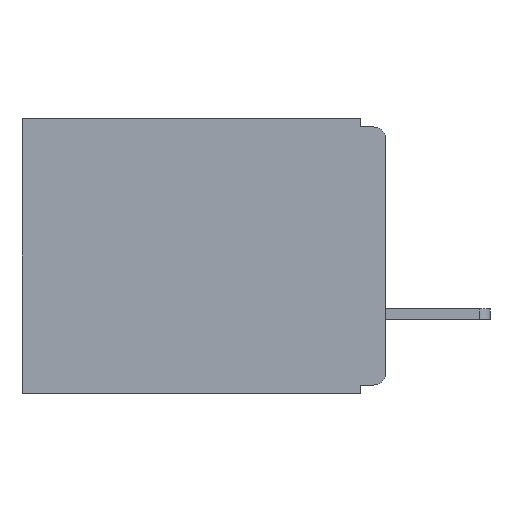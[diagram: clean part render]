
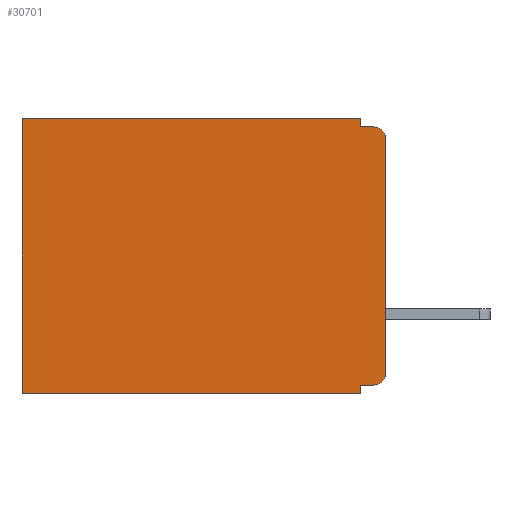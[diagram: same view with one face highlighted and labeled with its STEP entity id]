
A CAD part, left-side view. The second image highlights one B-rep face of the part: STEP entity #30701.
In plain terms, the highlighted planar face has unit normal (-1, 0, 0).
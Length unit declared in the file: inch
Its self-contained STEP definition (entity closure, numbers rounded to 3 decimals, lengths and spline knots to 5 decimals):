
#264 = VERTEX_POINT ( 'NONE', #18152 ) ;
#410 = LINE ( 'NONE', #27130, #25650 ) ;
#534 = ORIENTED_EDGE ( 'NONE', *, *, #4870, .F. ) ;
#1173 = FACE_OUTER_BOUND ( 'NONE', #26101, .T. ) ;
#1331 = ORIENTED_EDGE ( 'NONE', *, *, #5463, .F. ) ;
#1792 = AXIS2_PLACEMENT_3D ( 'NONE', #12589, #29337, #15085 ) ;
#1932 = VERTEX_POINT ( 'NONE', #24491 ) ;
#1987 = VERTEX_POINT ( 'NONE', #24394 ) ;
#2111 = LINE ( 'NONE', #21609, #7904 ) ;
#2284 = ORIENTED_EDGE ( 'NONE', *, *, #25020, .T. ) ;
#2735 = VECTOR ( 'NONE', #19983, 39.37008 ) ;
#3111 = ORIENTED_EDGE ( 'NONE', *, *, #28612, .T. ) ;
#3761 = DIRECTION ( 'NONE',  ( 0., 0., -1. ) ) ;
#3838 = ORIENTED_EDGE ( 'NONE', *, *, #11249, .F. ) ;
#4196 = DIRECTION ( 'NONE',  ( 0., -1., 0. ) ) ;
#4428 = DIRECTION ( 'NONE',  ( 0., 0., -1. ) ) ;
#4479 = CARTESIAN_POINT ( 'NONE',  ( 0.3, 0., -0.305 ) ) ;
#4870 = EDGE_CURVE ( 'NONE', #17214, #27444, #29079, .T. ) ;
#5152 = CARTESIAN_POINT ( 'NONE',  ( 0.3, 0., -0.32 ) ) ;
#5463 = EDGE_CURVE ( 'NONE', #6183, #6926, #17572, .T. ) ;
#5671 = CARTESIAN_POINT ( 'NONE',  ( 0.3, 0.437, -0.33 ) ) ;
#5699 = ORIENTED_EDGE ( 'NONE', *, *, #7581, .F. ) ;
#6183 = VERTEX_POINT ( 'NONE', #15034 ) ;
#6699 = ORIENTED_EDGE ( 'NONE', *, *, #14913, .T. ) ;
#6926 = VERTEX_POINT ( 'NONE', #8152 ) ;
#7234 = ORIENTED_EDGE ( 'NONE', *, *, #10860, .F. ) ;
#7368 = EDGE_CURVE ( 'NONE', #17056, #27444, #7726, .T. ) ;
#7581 = EDGE_CURVE ( 'NONE', #1987, #264, #21901, .T. ) ;
#7591 = ORIENTED_EDGE ( 'NONE', *, *, #11203, .F. ) ;
#7726 = CIRCLE ( 'NONE', #21765, 0.015 ) ;
#7904 = VECTOR ( 'NONE', #9402, 39.37008 ) ;
#8152 = CARTESIAN_POINT ( 'NONE',  ( 0.3, 0.015, -0.01 ) ) ;
#8206 = ORIENTED_EDGE ( 'NONE', *, *, #7368, .T. ) ;
#8566 = LINE ( 'NONE', #5152, #2735 ) ;
#9402 = DIRECTION ( 'NONE',  ( 0., 1., 0. ) ) ;
#10323 = VERTEX_POINT ( 'NONE', #28539 ) ;
#10860 = EDGE_CURVE ( 'NONE', #1932, #1987, #24191, .T. ) ;
#10916 = DIRECTION ( 'NONE',  ( 0., 0., -1. ) ) ;
#11162 = DIRECTION ( 'NONE',  ( -1., 0., 0. ) ) ;
#11203 = EDGE_CURVE ( 'NONE', #17056, #1932, #8566, .T. ) ;
#11249 = EDGE_CURVE ( 'NONE', #25748, #6183, #410, .T. ) ;
#11384 = CARTESIAN_POINT ( 'NONE',  ( 0.3, 0.015, -0.305 ) ) ;
#12258 = CARTESIAN_POINT ( 'NONE',  ( 0.3, 0.015, -0.32 ) ) ;
#12589 = CARTESIAN_POINT ( 'NONE',  ( 0.3, 0.015, -0.025 ) ) ;
#12863 = CARTESIAN_POINT ( 'NONE',  ( 0.3, 0.031, 0. ) ) ;
#12900 = CARTESIAN_POINT ( 'NONE',  ( 0.3, 0., -0.025 ) ) ;
#14736 = VECTOR ( 'NONE', #30109, 39.37008 ) ;
#14913 = EDGE_CURVE ( 'NONE', #10323, #264, #30010, .T. ) ;
#15034 = CARTESIAN_POINT ( 'NONE',  ( 0.3, 0.031, -0.01 ) ) ;
#15085 = DIRECTION ( 'NONE',  ( 0., 0., -1. ) ) ;
#16164 = CARTESIAN_POINT ( 'NONE',  ( 0.3, 0.031, -0.33 ) ) ;
#16817 = VECTOR ( 'NONE', #4196, 39.37008 ) ;
#17056 = VERTEX_POINT ( 'NONE', #12258 ) ;
#17214 = VERTEX_POINT ( 'NONE', #12900 ) ;
#17572 = LINE ( 'NONE', #21020, #16817 ) ;
#17910 = VECTOR ( 'NONE', #3761, 39.37008 ) ;
#18152 = CARTESIAN_POINT ( 'NONE',  ( 0.3, 0.437, -0.33 ) ) ;
#19276 = DIRECTION ( 'NONE',  ( 1., 0., 0. ) ) ;
#19983 = DIRECTION ( 'NONE',  ( 0., 1., 0. ) ) ;
#20176 = DIRECTION ( 'NONE',  ( 0., 0., -1. ) ) ;
#20482 = DIRECTION ( 'NONE',  ( 0., 0., -1. ) ) ;
#20622 = VECTOR ( 'NONE', #29097, 39.37008 ) ;
#21020 = CARTESIAN_POINT ( 'NONE',  ( 0.3, 0., -0.01 ) ) ;
#21609 = CARTESIAN_POINT ( 'NONE',  ( 0.3, 0., 0. ) ) ;
#21765 = AXIS2_PLACEMENT_3D ( 'NONE', #11384, #11162, #10916 ) ;
#21901 = LINE ( 'NONE', #30100, #14736 ) ;
#21959 = CIRCLE ( 'NONE', #1792, 0.015 ) ;
#23759 = VECTOR ( 'NONE', #20482, 39.37008 ) ;
#24191 = LINE ( 'NONE', #16164, #17910 ) ;
#24394 = CARTESIAN_POINT ( 'NONE',  ( 0.3, 0.031, -0.33 ) ) ;
#24491 = CARTESIAN_POINT ( 'NONE',  ( 0.3, 0.031, -0.32 ) ) ;
#25020 = EDGE_CURVE ( 'NONE', #17214, #6926, #21959, .T. ) ;
#25650 = VECTOR ( 'NONE', #20176, 39.37008 ) ;
#25748 = VERTEX_POINT ( 'NONE', #12863 ) ;
#26101 = EDGE_LOOP ( 'NONE', ( #534, #2284, #1331, #3838, #3111, #6699, #5699, #7234, #7591, #8206 ) ) ;
#26258 = PLANE ( 'NONE',  #27581 ) ;
#27130 = CARTESIAN_POINT ( 'NONE',  ( 0.3, 0.031, 0. ) ) ;
#27444 = VERTEX_POINT ( 'NONE', #4479 ) ;
#27581 = AXIS2_PLACEMENT_3D ( 'NONE', #30954, #19276, #4428 ) ;
#28539 = CARTESIAN_POINT ( 'NONE',  ( 0.3, 0.437, 0. ) ) ;
#28612 = EDGE_CURVE ( 'NONE', #25748, #10323, #2111, .T. ) ;
#29079 = LINE ( 'NONE', #30536, #20622 ) ;
#29097 = DIRECTION ( 'NONE',  ( 0., 0., -1. ) ) ;
#29337 = DIRECTION ( 'NONE',  ( -1., 0., 0. ) ) ;
#30010 = LINE ( 'NONE', #5671, #23759 ) ;
#30100 = CARTESIAN_POINT ( 'NONE',  ( 0.3, 0., -0.33 ) ) ;
#30109 = DIRECTION ( 'NONE',  ( 0., 1., 0. ) ) ;
#30536 = CARTESIAN_POINT ( 'NONE',  ( 0.3, 0., -0.33 ) ) ;
#30701 = ADVANCED_FACE ( 'NONE', ( #1173 ), #26258, .F. ) ;
#30954 = CARTESIAN_POINT ( 'NONE',  ( 0.3, 0., -0.33 ) ) ;
